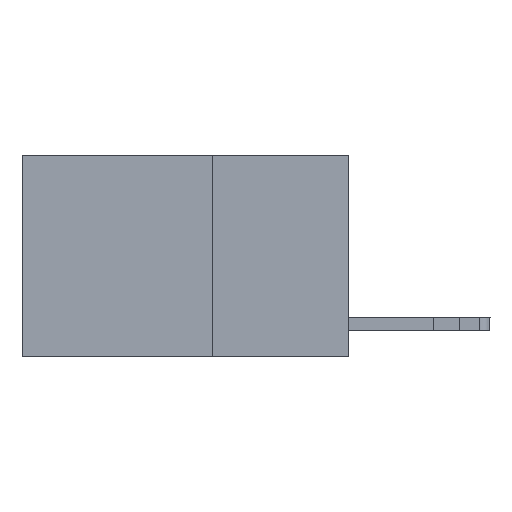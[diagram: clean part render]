
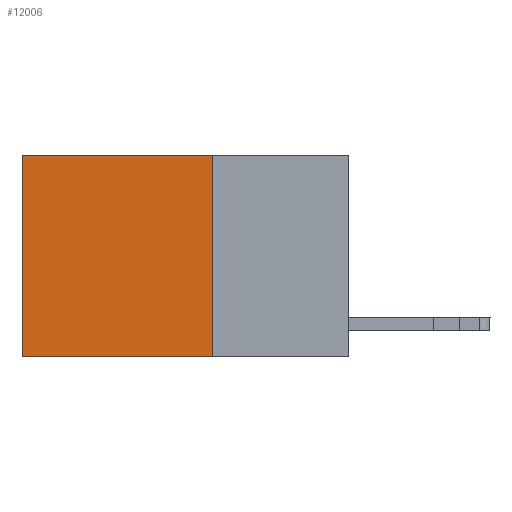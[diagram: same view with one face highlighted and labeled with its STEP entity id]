
A CAD part, left-side view. The second image highlights one B-rep face of the part: STEP entity #12006.
In plain terms, the highlighted planar face has unit normal (-1, 0, 0).
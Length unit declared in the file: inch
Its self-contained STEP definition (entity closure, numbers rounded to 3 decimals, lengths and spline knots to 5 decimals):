
#202 = DIRECTION ( 'NONE',  ( 0., 1., 0. ) ) ;
#262 = DIRECTION ( 'NONE',  ( 0., 0., -1. ) ) ;
#277 = CARTESIAN_POINT ( 'NONE',  ( 0.2625, 0.25, -0.37 ) ) ;
#1567 = VERTEX_POINT ( 'NONE', #10841 ) ;
#2152 = VECTOR ( 'NONE', #202, 39.37008 ) ;
#2665 = EDGE_CURVE ( 'NONE', #9515, #12345, #12909, .T. ) ;
#2799 = CARTESIAN_POINT ( 'NONE',  ( 0.2625, 0.25, 0. ) ) ;
#2922 = LINE ( 'NONE', #5811, #13057 ) ;
#3296 = CARTESIAN_POINT ( 'NONE',  ( 0.2625, 0.25, 0. ) ) ;
#3686 = CARTESIAN_POINT ( 'NONE',  ( 0.2625, 0.25, -0.37 ) ) ;
#4160 = CARTESIAN_POINT ( 'NONE',  ( 0.2625, 0.25, 0. ) ) ;
#4512 = EDGE_CURVE ( 'NONE', #12345, #9272, #11451, .T. ) ;
#5711 = AXIS2_PLACEMENT_3D ( 'NONE', #4160, #9217, #262 ) ;
#5811 = CARTESIAN_POINT ( 'NONE',  ( 0.2625, 0.6, 0. ) ) ;
#5965 = DIRECTION ( 'NONE',  ( 0., 1., 0. ) ) ;
#6050 = ORIENTED_EDGE ( 'NONE', *, *, #12739, .T. ) ;
#6757 = DIRECTION ( 'NONE',  ( 0., 0., -1. ) ) ;
#7019 = DIRECTION ( 'NONE',  ( 0., 0., -1. ) ) ;
#7560 = CARTESIAN_POINT ( 'NONE',  ( 0.2625, 0.6, -0.37 ) ) ;
#7769 = CARTESIAN_POINT ( 'NONE',  ( 0.2625, 0.25, 0. ) ) ;
#9217 = DIRECTION ( 'NONE',  ( 1., 0., 0. ) ) ;
#9272 = VERTEX_POINT ( 'NONE', #7560 ) ;
#9515 = VERTEX_POINT ( 'NONE', #3296 ) ;
#9534 = ORIENTED_EDGE ( 'NONE', *, *, #9714, .T. ) ;
#9714 = EDGE_CURVE ( 'NONE', #9515, #1567, #11907, .T. ) ;
#9969 = VECTOR ( 'NONE', #5965, 39.37008 ) ;
#10290 = ORIENTED_EDGE ( 'NONE', *, *, #4512, .F. ) ;
#10413 = FACE_OUTER_BOUND ( 'NONE', #11024, .T. ) ;
#10841 = CARTESIAN_POINT ( 'NONE',  ( 0.2625, 0.6, 0. ) ) ;
#10991 = ORIENTED_EDGE ( 'NONE', *, *, #2665, .F. ) ;
#11024 = EDGE_LOOP ( 'NONE', ( #6050, #10290, #10991, #9534 ) ) ;
#11451 = LINE ( 'NONE', #277, #2152 ) ;
#11907 = LINE ( 'NONE', #2799, #9969 ) ;
#12006 = ADVANCED_FACE ( 'NONE', ( #10413 ), #12513, .F. ) ;
#12345 = VERTEX_POINT ( 'NONE', #3686 ) ;
#12513 = PLANE ( 'NONE',  #5711 ) ;
#12739 = EDGE_CURVE ( 'NONE', #1567, #9272, #2922, .T. ) ;
#12909 = LINE ( 'NONE', #7769, #12947 ) ;
#12947 = VECTOR ( 'NONE', #6757, 39.37008 ) ;
#13057 = VECTOR ( 'NONE', #7019, 39.37008 ) ;
